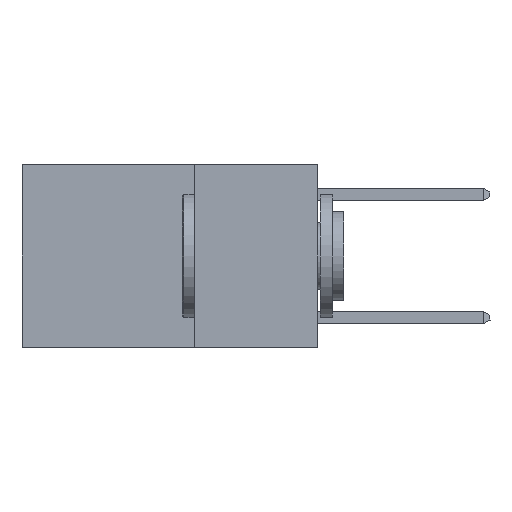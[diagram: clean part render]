
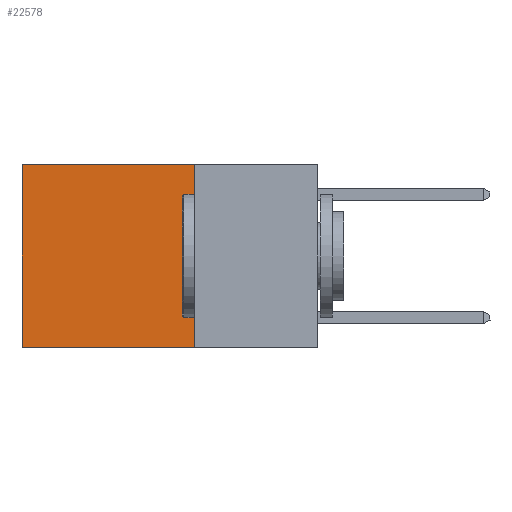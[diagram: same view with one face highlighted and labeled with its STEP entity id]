
A CAD part, left-side view. The second image highlights one B-rep face of the part: STEP entity #22578.
In plain terms, the highlighted planar face has unit normal (-1, 0, 0).
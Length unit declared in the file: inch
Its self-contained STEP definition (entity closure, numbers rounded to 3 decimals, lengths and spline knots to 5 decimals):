
#998 = CARTESIAN_POINT ( 'NONE',  ( 0.2625, 0.25, 0. ) ) ;
#1021 = ORIENTED_EDGE ( 'NONE', *, *, #2605, .F. ) ;
#2231 = EDGE_CURVE ( 'NONE', #23452, #9406, #15396, .T. ) ;
#2605 = EDGE_CURVE ( 'NONE', #23452, #9863, #24706, .T. ) ;
#3229 = PLANE ( 'NONE',  #11213 ) ;
#3626 = VECTOR ( 'NONE', #10877, 39.37008 ) ;
#5139 = FACE_OUTER_BOUND ( 'NONE', #7659, .T. ) ;
#5171 = VECTOR ( 'NONE', #20304, 39.37008 ) ;
#5531 = DIRECTION ( 'NONE',  ( 0., 0., -1. ) ) ;
#6401 = CARTESIAN_POINT ( 'NONE',  ( 0.2625, 0.25, -0.37 ) ) ;
#6894 = ORIENTED_EDGE ( 'NONE', *, *, #11318, .F. ) ;
#7659 = EDGE_LOOP ( 'NONE', ( #26404, #6894, #1021, #18954 ) ) ;
#7964 = LINE ( 'NONE', #26722, #12436 ) ;
#8686 = CARTESIAN_POINT ( 'NONE',  ( 0.2625, 0.25, 0. ) ) ;
#9406 = VERTEX_POINT ( 'NONE', #11832 ) ;
#9863 = VERTEX_POINT ( 'NONE', #6401 ) ;
#10877 = DIRECTION ( 'NONE',  ( 0., 1., 0. ) ) ;
#11213 = AXIS2_PLACEMENT_3D ( 'NONE', #27540, #18779, #5531 ) ;
#11318 = EDGE_CURVE ( 'NONE', #9863, #24667, #7964, .T. ) ;
#11394 = EDGE_CURVE ( 'NONE', #9406, #24667, #22780, .T. ) ;
#11832 = CARTESIAN_POINT ( 'NONE',  ( 0.2625, 0.6, 0. ) ) ;
#12436 = VECTOR ( 'NONE', #17832, 39.37008 ) ;
#15396 = LINE ( 'NONE', #8686, #3626 ) ;
#16485 = DIRECTION ( 'NONE',  ( 0., 0., -1. ) ) ;
#17832 = DIRECTION ( 'NONE',  ( 0., 1., 0. ) ) ;
#18108 = CARTESIAN_POINT ( 'NONE',  ( 0.2625, 0.6, 0. ) ) ;
#18779 = DIRECTION ( 'NONE',  ( 1., 0., 0. ) ) ;
#18814 = VECTOR ( 'NONE', #16485, 39.37008 ) ;
#18954 = ORIENTED_EDGE ( 'NONE', *, *, #2231, .T. ) ;
#20304 = DIRECTION ( 'NONE',  ( 0., 0., -1. ) ) ;
#21590 = CARTESIAN_POINT ( 'NONE',  ( 0.2625, 0.25, 0. ) ) ;
#22525 = CARTESIAN_POINT ( 'NONE',  ( 0.2625, 0.6, -0.37 ) ) ;
#22578 = ADVANCED_FACE ( 'NONE', ( #5139 ), #3229, .F. ) ;
#22780 = LINE ( 'NONE', #18108, #5171 ) ;
#23452 = VERTEX_POINT ( 'NONE', #21590 ) ;
#24667 = VERTEX_POINT ( 'NONE', #22525 ) ;
#24706 = LINE ( 'NONE', #998, #18814 ) ;
#26404 = ORIENTED_EDGE ( 'NONE', *, *, #11394, .T. ) ;
#26722 = CARTESIAN_POINT ( 'NONE',  ( 0.2625, 0.25, -0.37 ) ) ;
#27540 = CARTESIAN_POINT ( 'NONE',  ( 0.2625, 0.25, 0. ) ) ;
